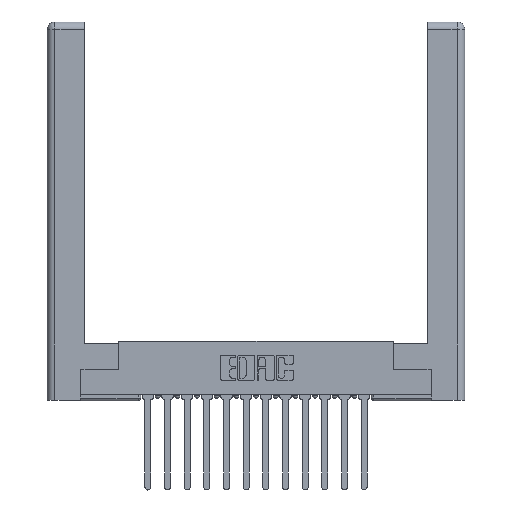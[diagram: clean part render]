
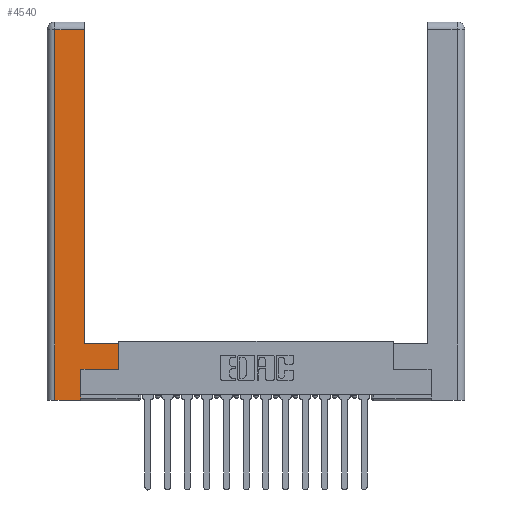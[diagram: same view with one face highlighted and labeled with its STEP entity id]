
A CAD part, top view. The second image highlights one B-rep face of the part: STEP entity #4540.
In plain terms, the highlighted planar face has unit normal (0, 0, 1).
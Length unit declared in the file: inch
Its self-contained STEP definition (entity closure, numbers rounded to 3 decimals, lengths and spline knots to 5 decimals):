
#103 = LINE ( 'NONE', #9098, #11945 ) ;
#251 = ORIENTED_EDGE ( 'NONE', *, *, #2470, .T. ) ;
#613 = ORIENTED_EDGE ( 'NONE', *, *, #14427, .T. ) ;
#656 = EDGE_CURVE ( 'NONE', #5527, #8194, #9229, .T. ) ;
#1063 = CARTESIAN_POINT ( 'NONE',  ( 0.265, 0., 0. ) ) ;
#1834 = VERTEX_POINT ( 'NONE', #10082 ) ;
#1945 = FACE_OUTER_BOUND ( 'NONE', #7148, .T. ) ;
#2357 = VECTOR ( 'NONE', #13877, 39.37008 ) ;
#2470 = EDGE_CURVE ( 'NONE', #3560, #5527, #5198, .T. ) ;
#2563 = CARTESIAN_POINT ( 'NONE',  ( 0.295, 0.45, 0. ) ) ;
#2972 = DIRECTION ( 'NONE',  ( 0., -1., 0. ) ) ;
#3336 = DIRECTION ( 'NONE',  ( 0., 1., 0. ) ) ;
#3560 = VERTEX_POINT ( 'NONE', #6545 ) ;
#3617 = EDGE_CURVE ( 'NONE', #1834, #14035, #4611, .T. ) ;
#3908 = ORIENTED_EDGE ( 'NONE', *, *, #13064, .T. ) ;
#3953 = VERTEX_POINT ( 'NONE', #1063 ) ;
#4540 = ADVANCED_FACE ( 'NONE', ( #1945 ), #15062, .F. ) ;
#4611 = LINE ( 'NONE', #5401, #11008 ) ;
#4725 = CARTESIAN_POINT ( 'NONE',  ( 0.565, 0.45, 0. ) ) ;
#4807 = EDGE_CURVE ( 'NONE', #8194, #6141, #7773, .T. ) ;
#4869 = CARTESIAN_POINT ( 'NONE',  ( 0., 0., 0. ) ) ;
#5198 = LINE ( 'NONE', #12749, #2357 ) ;
#5215 = LINE ( 'NONE', #11728, #11971 ) ;
#5401 = CARTESIAN_POINT ( 'NONE',  ( 0.0615, 0., 0. ) ) ;
#5527 = VERTEX_POINT ( 'NONE', #6540 ) ;
#5888 = VERTEX_POINT ( 'NONE', #7301 ) ;
#6141 = VERTEX_POINT ( 'NONE', #2563 ) ;
#6342 = CARTESIAN_POINT ( 'NONE',  ( 0.295, 0.45, 0. ) ) ;
#6540 = CARTESIAN_POINT ( 'NONE',  ( 0.565, 0.245, 0. ) ) ;
#6545 = CARTESIAN_POINT ( 'NONE',  ( 0.265, 0.245, 0. ) ) ;
#7148 = EDGE_LOOP ( 'NONE', ( #613, #10584, #10327, #15816, #3908, #251, #7519, #13031 ) ) ;
#7265 = VECTOR ( 'NONE', #14542, 39.37008 ) ;
#7301 = CARTESIAN_POINT ( 'NONE',  ( 0.295, 2.94, 0. ) ) ;
#7499 = DIRECTION ( 'NONE',  ( 0., 0., -1. ) ) ;
#7519 = ORIENTED_EDGE ( 'NONE', *, *, #656, .T. ) ;
#7773 = LINE ( 'NONE', #6342, #16341 ) ;
#8194 = VERTEX_POINT ( 'NONE', #4725 ) ;
#9035 = DIRECTION ( 'NONE',  ( -1., 0., 0. ) ) ;
#9098 = CARTESIAN_POINT ( 'NONE',  ( 0.0615, 2.94, 0. ) ) ;
#9229 = LINE ( 'NONE', #13679, #15610 ) ;
#10082 = CARTESIAN_POINT ( 'NONE',  ( 0.0615, 2.94, 0. ) ) ;
#10327 = ORIENTED_EDGE ( 'NONE', *, *, #3617, .T. ) ;
#10584 = ORIENTED_EDGE ( 'NONE', *, *, #15476, .T. ) ;
#10625 = LINE ( 'NONE', #12940, #7265 ) ;
#10984 = CARTESIAN_POINT ( 'NONE',  ( 0.0615, 0., 0. ) ) ;
#11008 = VECTOR ( 'NONE', #2972, 39.37008 ) ;
#11058 = DIRECTION ( 'NONE',  ( -1., 0., 0. ) ) ;
#11728 = CARTESIAN_POINT ( 'NONE',  ( 0.295, 3., 0. ) ) ;
#11788 = DIRECTION ( 'NONE',  ( 0., 1., 0. ) ) ;
#11830 = LINE ( 'NONE', #15379, #12032 ) ;
#11945 = VECTOR ( 'NONE', #12997, 39.37008 ) ;
#11971 = VECTOR ( 'NONE', #13034, 39.37008 ) ;
#12032 = VECTOR ( 'NONE', #11788, 39.37008 ) ;
#12593 = EDGE_CURVE ( 'NONE', #14035, #3953, #10625, .T. ) ;
#12607 = AXIS2_PLACEMENT_3D ( 'NONE', #4869, #7499, #11058 ) ;
#12749 = CARTESIAN_POINT ( 'NONE',  ( 0.565, 0.245, 0. ) ) ;
#12940 = CARTESIAN_POINT ( 'NONE',  ( 0.265, 0., 0. ) ) ;
#12997 = DIRECTION ( 'NONE',  ( -1., 0., 0. ) ) ;
#13031 = ORIENTED_EDGE ( 'NONE', *, *, #4807, .T. ) ;
#13034 = DIRECTION ( 'NONE',  ( 0., 1., 0. ) ) ;
#13064 = EDGE_CURVE ( 'NONE', #3953, #3560, #11830, .T. ) ;
#13679 = CARTESIAN_POINT ( 'NONE',  ( 0.565, 0.45, 0. ) ) ;
#13877 = DIRECTION ( 'NONE',  ( 1., 0., 0. ) ) ;
#14035 = VERTEX_POINT ( 'NONE', #10984 ) ;
#14427 = EDGE_CURVE ( 'NONE', #6141, #5888, #5215, .T. ) ;
#14542 = DIRECTION ( 'NONE',  ( 1., 0., 0. ) ) ;
#15062 = PLANE ( 'NONE',  #12607 ) ;
#15379 = CARTESIAN_POINT ( 'NONE',  ( 0.265, 0.245, 0. ) ) ;
#15476 = EDGE_CURVE ( 'NONE', #5888, #1834, #103, .T. ) ;
#15610 = VECTOR ( 'NONE', #3336, 39.37008 ) ;
#15816 = ORIENTED_EDGE ( 'NONE', *, *, #12593, .T. ) ;
#16341 = VECTOR ( 'NONE', #9035, 39.37008 ) ;
